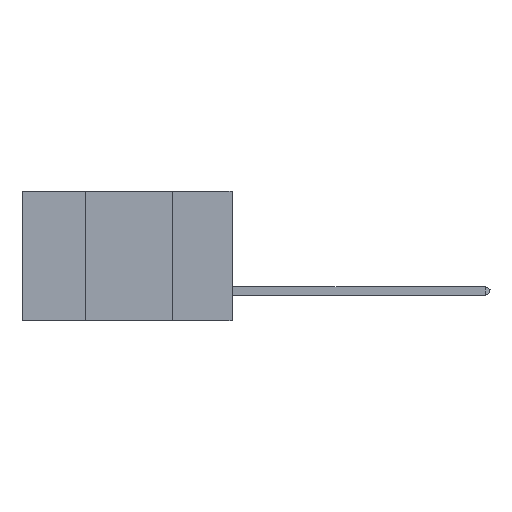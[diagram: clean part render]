
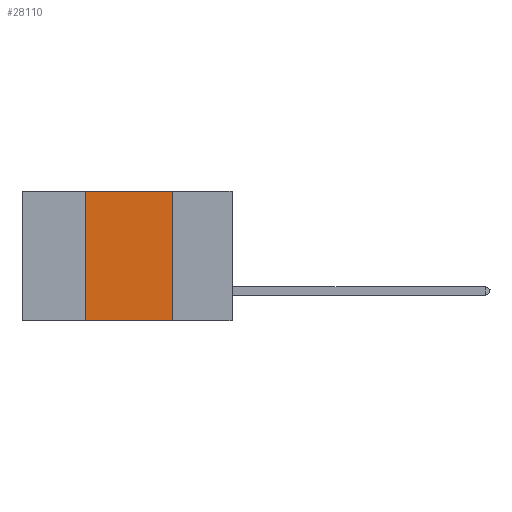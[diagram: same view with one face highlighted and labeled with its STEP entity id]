
A CAD part, left-side view. The second image highlights one B-rep face of the part: STEP entity #28110.
In plain terms, the highlighted planar face has unit normal (-1, 0, 0).
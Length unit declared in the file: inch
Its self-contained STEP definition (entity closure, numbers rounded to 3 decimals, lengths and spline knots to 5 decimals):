
#1855 = ORIENTED_EDGE ( 'NONE', *, *, #7002, .T. ) ;
#4202 = EDGE_CURVE ( 'NONE', #36546, #26861, #22850, .T. ) ;
#6017 = VECTOR ( 'NONE', #24633, 39.37008 ) ;
#6681 = CARTESIAN_POINT ( 'NONE',  ( 0., 0.42, -0.37 ) ) ;
#6925 = FACE_OUTER_BOUND ( 'NONE', #12116, .T. ) ;
#7002 = EDGE_CURVE ( 'NONE', #20804, #7026, #7087, .T. ) ;
#7026 = VERTEX_POINT ( 'NONE', #28783 ) ;
#7087 = LINE ( 'NONE', #17782, #15113 ) ;
#7357 = AXIS2_PLACEMENT_3D ( 'NONE', #13003, #20144, #33279 ) ;
#7812 = VECTOR ( 'NONE', #30428, 39.37008 ) ;
#12116 = EDGE_LOOP ( 'NONE', ( #42324, #32076, #19910, #1855 ) ) ;
#13003 = CARTESIAN_POINT ( 'NONE',  ( 0., 0.6, 0. ) ) ;
#15113 = VECTOR ( 'NONE', #17504, 39.37008 ) ;
#17504 = DIRECTION ( 'NONE',  ( 0., -1., 0. ) ) ;
#17782 = CARTESIAN_POINT ( 'NONE',  ( 0., 0.6, -0.37 ) ) ;
#18436 = DIRECTION ( 'NONE',  ( 0., -1., 0. ) ) ;
#19531 = EDGE_CURVE ( 'NONE', #20804, #36546, #39561, .T. ) ;
#19605 = VECTOR ( 'NONE', #18436, 39.37008 ) ;
#19910 = ORIENTED_EDGE ( 'NONE', *, *, #19531, .F. ) ;
#20144 = DIRECTION ( 'NONE',  ( 1., 0., 0. ) ) ;
#20804 = VERTEX_POINT ( 'NONE', #6681 ) ;
#22850 = LINE ( 'NONE', #41925, #19605 ) ;
#24633 = DIRECTION ( 'NONE',  ( 0., 0., -1. ) ) ;
#25624 = CARTESIAN_POINT ( 'NONE',  ( 0., 0.17, 0. ) ) ;
#26861 = VERTEX_POINT ( 'NONE', #25624 ) ;
#27260 = CARTESIAN_POINT ( 'NONE',  ( 0., 0.42, 0. ) ) ;
#28110 = ADVANCED_FACE ( 'NONE', ( #6925 ), #33759, .F. ) ;
#28783 = CARTESIAN_POINT ( 'NONE',  ( 0., 0.17, -0.37 ) ) ;
#30428 = DIRECTION ( 'NONE',  ( 0., 0., 1. ) ) ;
#32076 = ORIENTED_EDGE ( 'NONE', *, *, #4202, .F. ) ;
#33279 = DIRECTION ( 'NONE',  ( 0., 0., -1. ) ) ;
#33759 = PLANE ( 'NONE',  #7357 ) ;
#34572 = LINE ( 'NONE', #35696, #6017 ) ;
#35696 = CARTESIAN_POINT ( 'NONE',  ( 0., 0.17, 0. ) ) ;
#36546 = VERTEX_POINT ( 'NONE', #44428 ) ;
#39561 = LINE ( 'NONE', #27260, #7812 ) ;
#41925 = CARTESIAN_POINT ( 'NONE',  ( 0., 0.6, 0. ) ) ;
#42324 = ORIENTED_EDGE ( 'NONE', *, *, #43396, .F. ) ;
#43396 = EDGE_CURVE ( 'NONE', #26861, #7026, #34572, .T. ) ;
#44428 = CARTESIAN_POINT ( 'NONE',  ( 0., 0.42, 0. ) ) ;
